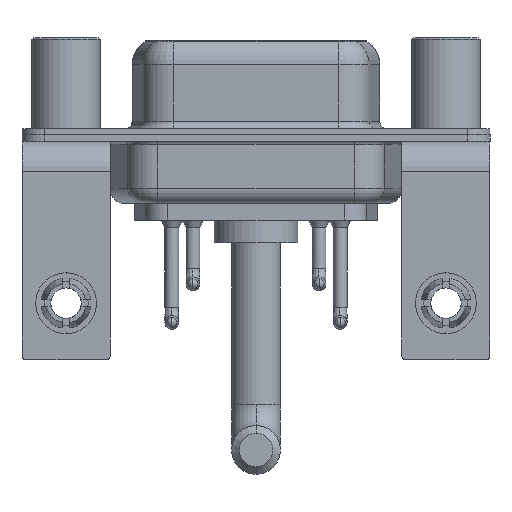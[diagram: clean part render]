
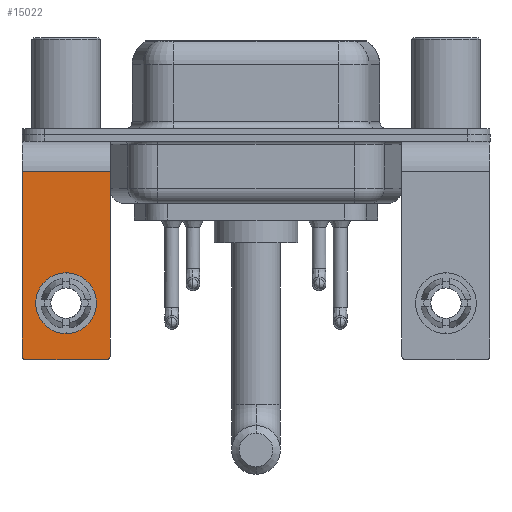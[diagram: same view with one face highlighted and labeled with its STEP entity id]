
A CAD part, front view. The second image highlights one B-rep face of the part: STEP entity #15022.
In plain terms, the highlighted planar face has unit normal (0, -1, 0).
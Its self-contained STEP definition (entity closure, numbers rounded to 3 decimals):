
#353 = EDGE_CURVE ( 'NONE', #844, #15397, #17440, .T. ) ;
#371 = DIRECTION ( 'NONE',  ( 0., 0., 1. ) ) ;
#553 = VECTOR ( 'NONE', #17228, 1000. ) ;
#844 = VERTEX_POINT ( 'NONE', #9766 ) ;
#1319 = VECTOR ( 'NONE', #9854, 1000. ) ;
#1375 = CARTESIAN_POINT ( 'NONE',  ( 0., -6.25, -9.07 ) ) ;
#1520 = DIRECTION ( 'NONE',  ( 0., 1., 0. ) ) ;
#1746 = DIRECTION ( 'NONE',  ( 0., 0., 1. ) ) ;
#1908 = AXIS2_PLACEMENT_3D ( 'NONE', #4468, #10597, #12398 ) ;
#2165 = VERTEX_POINT ( 'NONE', #16092 ) ;
#2187 = ORIENTED_EDGE ( 'NONE', *, *, #19522, .F. ) ;
#2841 = FACE_OUTER_BOUND ( 'NONE', #19295, .T. ) ;
#2898 = EDGE_CURVE ( 'NONE', #6300, #15802, #14387, .T. ) ;
#3239 = VECTOR ( 'NONE', #4306, 1000. ) ;
#3276 = CARTESIAN_POINT ( 'NONE',  ( 2.9, -6.25, -14.8 ) ) ;
#3339 = ORIENTED_EDGE ( 'NONE', *, *, #18060, .T. ) ;
#3405 = PLANE ( 'NONE',  #7292 ) ;
#3716 = CARTESIAN_POINT ( 'NONE',  ( 2.9, -6.25, -2.4 ) ) ;
#4103 = DIRECTION ( 'NONE',  ( 0., -1., 0. ) ) ;
#4306 = DIRECTION ( 'NONE',  ( 0., 0., -1. ) ) ;
#4468 = CARTESIAN_POINT ( 'NONE',  ( 2.65, -6.25, -14.55 ) ) ;
#5698 = AXIS2_PLACEMENT_3D ( 'NONE', #9715, #8108, #17029 ) ;
#5709 = LINE ( 'NONE', #6098, #3239 ) ;
#5714 = CARTESIAN_POINT ( 'NONE',  ( -2.65, -6.25, -14.55 ) ) ;
#5857 = VECTOR ( 'NONE', #17563, 1000. ) ;
#5941 = ORIENTED_EDGE ( 'NONE', *, *, #15612, .T. ) ;
#5975 = EDGE_CURVE ( 'NONE', #2165, #16851, #16027, .T. ) ;
#6098 = CARTESIAN_POINT ( 'NONE',  ( -2.9, -6.25, -2.4 ) ) ;
#6300 = VERTEX_POINT ( 'NONE', #7273 ) ;
#6495 = LINE ( 'NONE', #3276, #553 ) ;
#6676 = CARTESIAN_POINT ( 'NONE',  ( 2.9, -6.25, -2.4 ) ) ;
#7012 = ORIENTED_EDGE ( 'NONE', *, *, #15567, .F. ) ;
#7273 = CARTESIAN_POINT ( 'NONE',  ( -2.9, -6.25, -14.55 ) ) ;
#7292 = AXIS2_PLACEMENT_3D ( 'NONE', #14135, #1520, #371 ) ;
#7429 = VERTEX_POINT ( 'NONE', #6676 ) ;
#7898 = ORIENTED_EDGE ( 'NONE', *, *, #10431, .T. ) ;
#8108 = DIRECTION ( 'NONE',  ( 0., 1., 0. ) ) ;
#8204 = ORIENTED_EDGE ( 'NONE', *, *, #353, .T. ) ;
#8268 = ORIENTED_EDGE ( 'NONE', *, *, #2898, .T. ) ;
#8272 = CARTESIAN_POINT ( 'NONE',  ( 0., -6.25, -11.07 ) ) ;
#8804 = AXIS2_PLACEMENT_3D ( 'NONE', #8272, #11179, #1746 ) ;
#9715 = CARTESIAN_POINT ( 'NONE',  ( 0., -6.25, -11.07 ) ) ;
#9766 = CARTESIAN_POINT ( 'NONE',  ( 0., -6.25, -13.07 ) ) ;
#9854 = DIRECTION ( 'NONE',  ( 0., 0., -1. ) ) ;
#10431 = EDGE_CURVE ( 'NONE', #7429, #12384, #16259, .T. ) ;
#10597 = DIRECTION ( 'NONE',  ( 0., -1., 0. ) ) ;
#10785 = CARTESIAN_POINT ( 'NONE',  ( -2.9, -6.25, -2.4 ) ) ;
#11156 = CARTESIAN_POINT ( 'NONE',  ( 2.9, -6.25, -2.4 ) ) ;
#11179 = DIRECTION ( 'NONE',  ( 0., 1., 0. ) ) ;
#11788 = CIRCLE ( 'NONE', #5698, 2. ) ;
#12384 = VERTEX_POINT ( 'NONE', #10785 ) ;
#12398 = DIRECTION ( 'NONE',  ( 0., 0., 1. ) ) ;
#14111 = CARTESIAN_POINT ( 'NONE',  ( 2.9, -6.25, -14.55 ) ) ;
#14135 = CARTESIAN_POINT ( 'NONE',  ( 2.9, -6.25, -2.4 ) ) ;
#14387 = CIRCLE ( 'NONE', #15689, 0.25 ) ;
#14947 = DIRECTION ( 'NONE',  ( 0., 0., 1. ) ) ;
#15022 = ADVANCED_FACE ( 'NONE', ( #18191, #2841 ), #3405, .F. ) ;
#15397 = VERTEX_POINT ( 'NONE', #1375 ) ;
#15567 = EDGE_CURVE ( 'NONE', #2165, #15802, #6495, .T. ) ;
#15612 = EDGE_CURVE ( 'NONE', #15397, #844, #11788, .T. ) ;
#15689 = AXIS2_PLACEMENT_3D ( 'NONE', #5714, #4103, #14947 ) ;
#15802 = VERTEX_POINT ( 'NONE', #19033 ) ;
#16027 = CIRCLE ( 'NONE', #1908, 0.25 ) ;
#16092 = CARTESIAN_POINT ( 'NONE',  ( 2.65, -6.25, -14.8 ) ) ;
#16259 = LINE ( 'NONE', #3716, #5857 ) ;
#16851 = VERTEX_POINT ( 'NONE', #14111 ) ;
#17029 = DIRECTION ( 'NONE',  ( 0., 0., 1. ) ) ;
#17228 = DIRECTION ( 'NONE',  ( -1., 0., 0. ) ) ;
#17440 = CIRCLE ( 'NONE', #8804, 2. ) ;
#17527 = EDGE_LOOP ( 'NONE', ( #8204, #5941 ) ) ;
#17563 = DIRECTION ( 'NONE',  ( -1., 0., 0. ) ) ;
#18060 = EDGE_CURVE ( 'NONE', #12384, #6300, #5709, .T. ) ;
#18191 = FACE_BOUND ( 'NONE', #17527, .T. ) ;
#19033 = CARTESIAN_POINT ( 'NONE',  ( -2.65, -6.25, -14.8 ) ) ;
#19178 = LINE ( 'NONE', #11156, #1319 ) ;
#19295 = EDGE_LOOP ( 'NONE', ( #3339, #8268, #7012, #19751, #2187, #7898 ) ) ;
#19522 = EDGE_CURVE ( 'NONE', #7429, #16851, #19178, .T. ) ;
#19751 = ORIENTED_EDGE ( 'NONE', *, *, #5975, .T. ) ;
